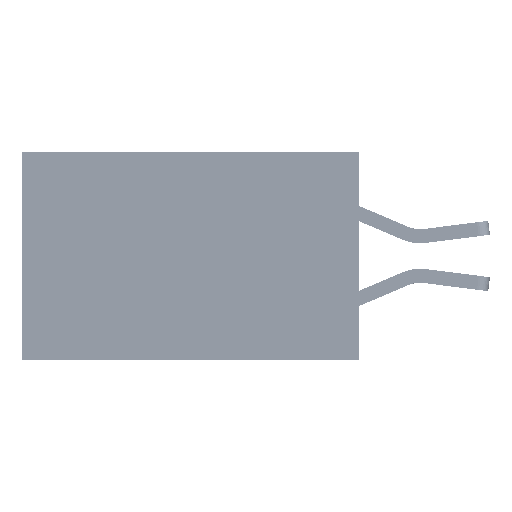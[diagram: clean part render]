
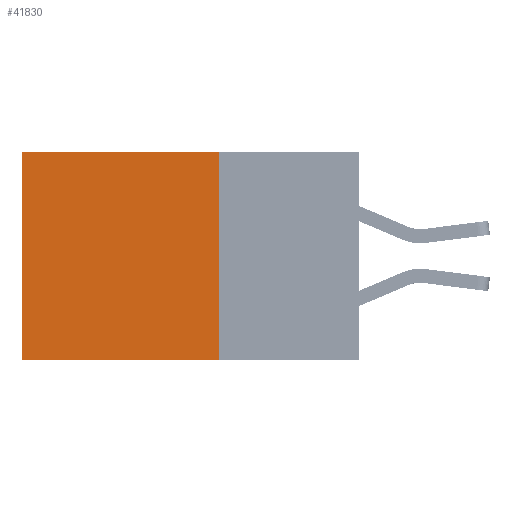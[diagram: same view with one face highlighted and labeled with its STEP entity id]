
A CAD part, left-side view. The second image highlights one B-rep face of the part: STEP entity #41830.
In plain terms, the highlighted planar face has unit normal (-1, 0, 0).
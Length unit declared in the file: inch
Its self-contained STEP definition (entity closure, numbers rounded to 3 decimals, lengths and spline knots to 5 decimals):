
#2122 = ORIENTED_EDGE ( 'NONE', *, *, #15075, .T. ) ;
#2902 = EDGE_CURVE ( 'NONE', #36210, #16278, #7422, .T. ) ;
#3310 = CARTESIAN_POINT ( 'NONE',  ( 0.2875, 0.25, -0.37 ) ) ;
#3541 = CARTESIAN_POINT ( 'NONE',  ( 0.2875, 0.25, 0. ) ) ;
#6482 = CARTESIAN_POINT ( 'NONE',  ( 0.2875, 0.6, 0. ) ) ;
#6877 = VECTOR ( 'NONE', #26483, 39.37008 ) ;
#7422 = LINE ( 'NONE', #42167, #32974 ) ;
#11532 = DIRECTION ( 'NONE',  ( 0., 1., 0. ) ) ;
#14262 = CARTESIAN_POINT ( 'NONE',  ( 0.2875, 0.6, 0. ) ) ;
#15075 = EDGE_CURVE ( 'NONE', #16278, #44828, #39986, .T. ) ;
#15521 = CARTESIAN_POINT ( 'NONE',  ( 0.2875, 0.6, -0.37 ) ) ;
#16278 = VERTEX_POINT ( 'NONE', #6482 ) ;
#16334 = DIRECTION ( 'NONE',  ( 0., 1., 0. ) ) ;
#16590 = ORIENTED_EDGE ( 'NONE', *, *, #2902, .T. ) ;
#17023 = VECTOR ( 'NONE', #16334, 39.37008 ) ;
#20442 = CARTESIAN_POINT ( 'NONE',  ( 0.2875, 0.25, 0. ) ) ;
#26483 = DIRECTION ( 'NONE',  ( 0., 0., -1. ) ) ;
#27910 = DIRECTION ( 'NONE',  ( 1., 0., 0. ) ) ;
#27921 = AXIS2_PLACEMENT_3D ( 'NONE', #20442, #27910, #47582 ) ;
#29637 = EDGE_LOOP ( 'NONE', ( #2122, #44307, #30868, #16590 ) ) ;
#30417 = DIRECTION ( 'NONE',  ( 0., 0., -1. ) ) ;
#30868 = ORIENTED_EDGE ( 'NONE', *, *, #32850, .F. ) ;
#32850 = EDGE_CURVE ( 'NONE', #36210, #33570, #40849, .T. ) ;
#32974 = VECTOR ( 'NONE', #11532, 39.37008 ) ;
#33570 = VERTEX_POINT ( 'NONE', #3310 ) ;
#36025 = PLANE ( 'NONE',  #27921 ) ;
#36210 = VERTEX_POINT ( 'NONE', #3541 ) ;
#38168 = VECTOR ( 'NONE', #30417, 39.37008 ) ;
#38249 = EDGE_CURVE ( 'NONE', #33570, #44828, #41332, .T. ) ;
#39986 = LINE ( 'NONE', #14262, #38168 ) ;
#40849 = LINE ( 'NONE', #49528, #6877 ) ;
#41332 = LINE ( 'NONE', #47432, #17023 ) ;
#41830 = ADVANCED_FACE ( 'NONE', ( #42817 ), #36025, .F. ) ;
#42167 = CARTESIAN_POINT ( 'NONE',  ( 0.2875, 0.25, 0. ) ) ;
#42817 = FACE_OUTER_BOUND ( 'NONE', #29637, .T. ) ;
#44307 = ORIENTED_EDGE ( 'NONE', *, *, #38249, .F. ) ;
#44828 = VERTEX_POINT ( 'NONE', #15521 ) ;
#47432 = CARTESIAN_POINT ( 'NONE',  ( 0.2875, 0.25, -0.37 ) ) ;
#47582 = DIRECTION ( 'NONE',  ( 0., 0., -1. ) ) ;
#49528 = CARTESIAN_POINT ( 'NONE',  ( 0.2875, 0.25, 0. ) ) ;
